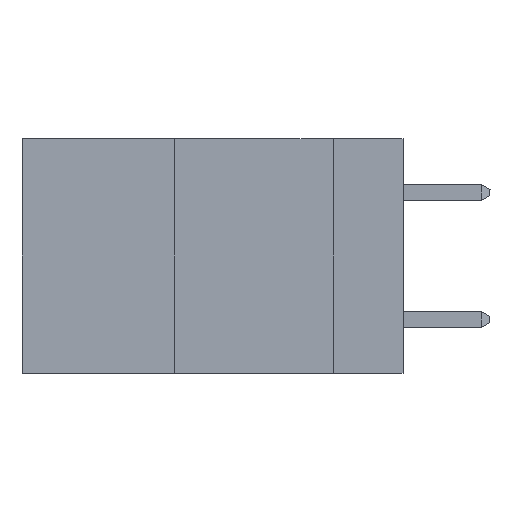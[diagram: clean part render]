
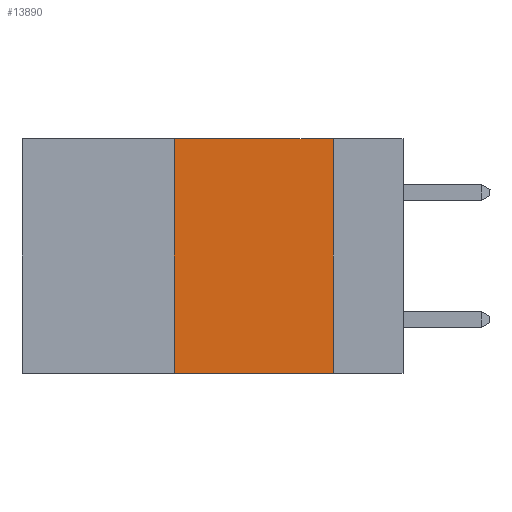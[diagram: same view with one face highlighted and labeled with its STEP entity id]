
A CAD part, left-side view. The second image highlights one B-rep face of the part: STEP entity #13890.
In plain terms, the highlighted planar face has unit normal (-1, 0, 0).
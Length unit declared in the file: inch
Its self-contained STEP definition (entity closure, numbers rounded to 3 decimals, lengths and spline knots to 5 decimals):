
#768 = EDGE_CURVE ( 'NONE', #17462, #4795, #7292, .T. ) ;
#2274 = CARTESIAN_POINT ( 'NONE',  ( 0., 0.11, -0.37 ) ) ;
#2750 = LINE ( 'NONE', #14002, #3237 ) ;
#2757 = CARTESIAN_POINT ( 'NONE',  ( 0., 0.36, -0.37 ) ) ;
#2932 = VECTOR ( 'NONE', #18764, 39.37008 ) ;
#3115 = EDGE_CURVE ( 'NONE', #7080, #4963, #20157, .T. ) ;
#3181 = ORIENTED_EDGE ( 'NONE', *, *, #14957, .F. ) ;
#3237 = VECTOR ( 'NONE', #4382, 39.37008 ) ;
#3259 = PLANE ( 'NONE',  #14848 ) ;
#3324 = ORIENTED_EDGE ( 'NONE', *, *, #10771, .F. ) ;
#4382 = DIRECTION ( 'NONE',  ( 0., 0., -1. ) ) ;
#4525 = ORIENTED_EDGE ( 'NONE', *, *, #768, .F. ) ;
#4795 = VERTEX_POINT ( 'NONE', #6781 ) ;
#4963 = VERTEX_POINT ( 'NONE', #2274 ) ;
#4977 = ORIENTED_EDGE ( 'NONE', *, *, #3115, .T. ) ;
#5136 = LINE ( 'NONE', #5411, #17756 ) ;
#5411 = CARTESIAN_POINT ( 'NONE',  ( 0., 0.36, 0. ) ) ;
#6569 = DIRECTION ( 'NONE',  ( 0., 0., -1. ) ) ;
#6781 = CARTESIAN_POINT ( 'NONE',  ( 0., 0.11, 0. ) ) ;
#7080 = VERTEX_POINT ( 'NONE', #2757 ) ;
#7292 = LINE ( 'NONE', #18700, #2932 ) ;
#8720 = DIRECTION ( 'NONE',  ( 0., -1., 0. ) ) ;
#8721 = VECTOR ( 'NONE', #8720, 39.37008 ) ;
#9196 = EDGE_LOOP ( 'NONE', ( #3181, #4525, #3324, #4977 ) ) ;
#10771 = EDGE_CURVE ( 'NONE', #7080, #17462, #5136, .T. ) ;
#11683 = FACE_OUTER_BOUND ( 'NONE', #9196, .T. ) ;
#13890 = ADVANCED_FACE ( 'NONE', ( #11683 ), #3259, .F. ) ;
#14002 = CARTESIAN_POINT ( 'NONE',  ( 0., 0.11, 0. ) ) ;
#14500 = CARTESIAN_POINT ( 'NONE',  ( 0., 0.6, 0. ) ) ;
#14848 = AXIS2_PLACEMENT_3D ( 'NONE', #14500, #16036, #6569 ) ;
#14957 = EDGE_CURVE ( 'NONE', #4795, #4963, #2750, .T. ) ;
#16036 = DIRECTION ( 'NONE',  ( 1., 0., 0. ) ) ;
#16047 = CARTESIAN_POINT ( 'NONE',  ( 0., 0.36, 0. ) ) ;
#17462 = VERTEX_POINT ( 'NONE', #16047 ) ;
#17756 = VECTOR ( 'NONE', #18040, 39.37008 ) ;
#18040 = DIRECTION ( 'NONE',  ( 0., 0., 1. ) ) ;
#18071 = CARTESIAN_POINT ( 'NONE',  ( 0., 0.6, -0.37 ) ) ;
#18700 = CARTESIAN_POINT ( 'NONE',  ( 0., 0.6, 0. ) ) ;
#18764 = DIRECTION ( 'NONE',  ( 0., -1., 0. ) ) ;
#20157 = LINE ( 'NONE', #18071, #8721 ) ;
